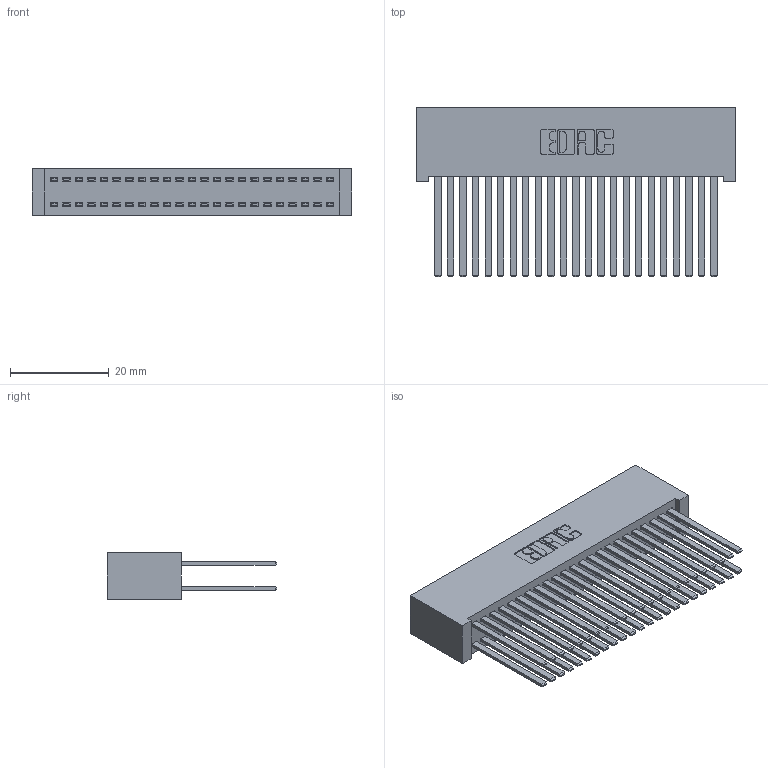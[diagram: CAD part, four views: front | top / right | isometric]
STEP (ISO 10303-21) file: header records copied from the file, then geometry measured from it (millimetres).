
FILE_DESCRIPTION (( 'STEP AP203' ), '1' );
FILE_NAME ('392-046-544-201.STEP', '2018-08-16T19:46:36', ( '' ), ( '' ), 'SwSTEP 2.0', 'SolidWorks 2016', '' );
FILE_SCHEMA (( 'CONFIG_CONTROL_DESIGN' ));
Length unit declared in the file: inch
Products named in the file (3): 342 Part_Lugless; 345-292-001_345-293-144; 392-046-544-201
Assembly tree (47 placements, depth 2):
  392-046-544-201
    342 Part_Lugless
    345-292-001_345-293-144  x46
Bounding box: 64.67 x 34.3 x 9.4 mm (x, y, z)
Volume: 6804.9 mm3; surface area: 12840.4 mm2
Topology: 47 solids, 47 shells, 2218 faces, 6577 edges, 4322 vertices
Faces by surface type: plane 1534, cylinder 684
Entity records: 16661 total; most frequent: CARTESIAN_POINT 2778, ORIENTED_EDGE 2714, DIRECTION 2397, EDGE_CURVE 1357, LINE 1241, VECTOR 1241, VERTEX_POINT 902, AXIS2_PLACEMENT_3D 578
